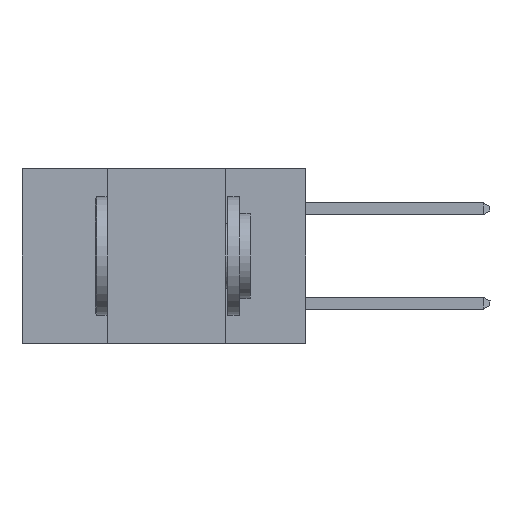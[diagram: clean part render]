
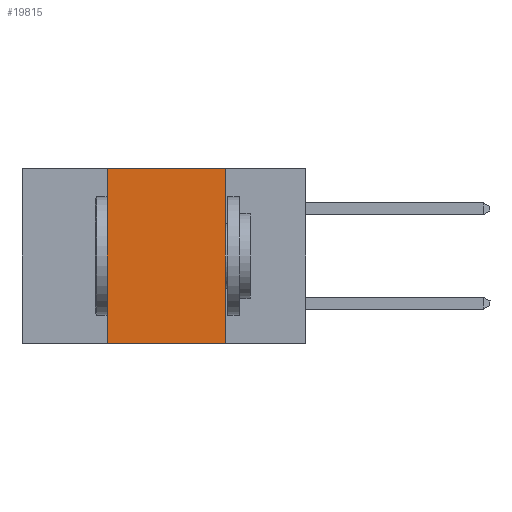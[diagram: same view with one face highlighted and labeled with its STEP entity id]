
A CAD part, left-side view. The second image highlights one B-rep face of the part: STEP entity #19815.
In plain terms, the highlighted planar face has unit normal (-1, 0, 0).
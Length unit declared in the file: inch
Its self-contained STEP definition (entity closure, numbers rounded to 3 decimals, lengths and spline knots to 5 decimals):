
#2723 = VECTOR ( 'NONE', #4237, 39.37008 ) ;
#4237 = DIRECTION ( 'NONE',  ( 0., -1., 0. ) ) ;
#5132 = EDGE_CURVE ( 'NONE', #6180, #25319, #33046, .T. ) ;
#6180 = VERTEX_POINT ( 'NONE', #17236 ) ;
#7106 = CARTESIAN_POINT ( 'NONE',  ( 0., 0.6, -0.37 ) ) ;
#9189 = EDGE_CURVE ( 'NONE', #25319, #17077, #13469, .T. ) ;
#9232 = DIRECTION ( 'NONE',  ( 1., 0., 0. ) ) ;
#10356 = CARTESIAN_POINT ( 'NONE',  ( 0., 0.17, -0.37 ) ) ;
#10379 = CARTESIAN_POINT ( 'NONE',  ( 0., 0.42, 0. ) ) ;
#11080 = EDGE_CURVE ( 'NONE', #22678, #17077, #19184, .T. ) ;
#13368 = ORIENTED_EDGE ( 'NONE', *, *, #32777, .F. ) ;
#13469 = LINE ( 'NONE', #21067, #22158 ) ;
#13819 = CARTESIAN_POINT ( 'NONE',  ( 0., 0.6, 0. ) ) ;
#14470 = LINE ( 'NONE', #10379, #33844 ) ;
#14603 = ORIENTED_EDGE ( 'NONE', *, *, #9189, .F. ) ;
#15610 = DIRECTION ( 'NONE',  ( 0., 0., 1. ) ) ;
#17077 = VERTEX_POINT ( 'NONE', #10356 ) ;
#17236 = CARTESIAN_POINT ( 'NONE',  ( 0., 0.42, 0. ) ) ;
#17675 = PLANE ( 'NONE',  #23262 ) ;
#19184 = LINE ( 'NONE', #7106, #2723 ) ;
#19815 = ADVANCED_FACE ( 'NONE', ( #20754 ), #17675, .F. ) ;
#20719 = VECTOR ( 'NONE', #32257, 39.37008 ) ;
#20754 = FACE_OUTER_BOUND ( 'NONE', #30245, .T. ) ;
#21067 = CARTESIAN_POINT ( 'NONE',  ( 0., 0.17, 0. ) ) ;
#21257 = ORIENTED_EDGE ( 'NONE', *, *, #5132, .F. ) ;
#22158 = VECTOR ( 'NONE', #23766, 39.37008 ) ;
#22678 = VERTEX_POINT ( 'NONE', #22946 ) ;
#22946 = CARTESIAN_POINT ( 'NONE',  ( 0., 0.42, -0.37 ) ) ;
#23262 = AXIS2_PLACEMENT_3D ( 'NONE', #28125, #9232, #27686 ) ;
#23766 = DIRECTION ( 'NONE',  ( 0., 0., -1. ) ) ;
#25319 = VERTEX_POINT ( 'NONE', #27007 ) ;
#27007 = CARTESIAN_POINT ( 'NONE',  ( 0., 0.17, 0. ) ) ;
#27686 = DIRECTION ( 'NONE',  ( 0., 0., -1. ) ) ;
#28125 = CARTESIAN_POINT ( 'NONE',  ( 0., 0.6, 0. ) ) ;
#30245 = EDGE_LOOP ( 'NONE', ( #14603, #21257, #13368, #30351 ) ) ;
#30351 = ORIENTED_EDGE ( 'NONE', *, *, #11080, .T. ) ;
#32257 = DIRECTION ( 'NONE',  ( 0., -1., 0. ) ) ;
#32777 = EDGE_CURVE ( 'NONE', #22678, #6180, #14470, .T. ) ;
#33046 = LINE ( 'NONE', #13819, #20719 ) ;
#33844 = VECTOR ( 'NONE', #15610, 39.37008 ) ;
